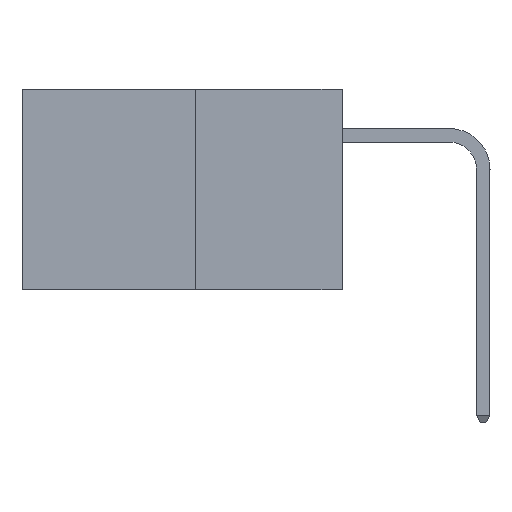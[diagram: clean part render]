
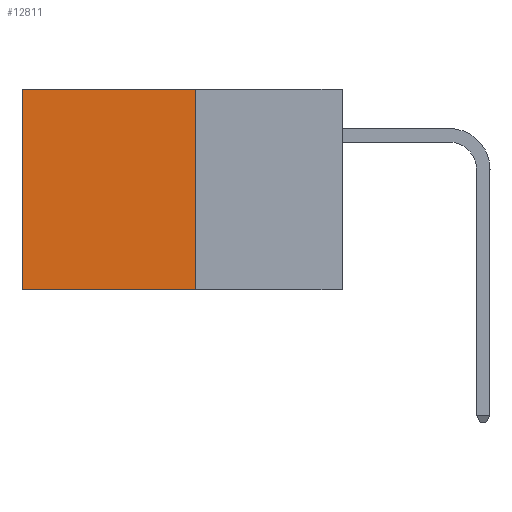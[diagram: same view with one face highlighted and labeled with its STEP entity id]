
A CAD part, left-side view. The second image highlights one B-rep face of the part: STEP entity #12811.
In plain terms, the highlighted planar face has unit normal (-1, 0, 0).
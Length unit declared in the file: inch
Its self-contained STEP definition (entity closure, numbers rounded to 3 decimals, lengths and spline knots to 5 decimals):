
#81 = VERTEX_POINT ( 'NONE', #2989 ) ;
#123 = EDGE_CURVE ( 'NONE', #5820, #247, #1685, .T. ) ;
#197 = CARTESIAN_POINT ( 'NONE',  ( 0.277, 0.59, -0.37 ) ) ;
#247 = VERTEX_POINT ( 'NONE', #4695 ) ;
#1388 = PLANE ( 'NONE',  #12118 ) ;
#1685 = LINE ( 'NONE', #8712, #4785 ) ;
#2610 = DIRECTION ( 'NONE',  ( 0., 0., -1. ) ) ;
#2716 = VECTOR ( 'NONE', #12440, 39.37008 ) ;
#2989 = CARTESIAN_POINT ( 'NONE',  ( 0.277, 0.59, 0. ) ) ;
#3419 = CARTESIAN_POINT ( 'NONE',  ( 0.277, 0.27, -0.37 ) ) ;
#4319 = EDGE_CURVE ( 'NONE', #13205, #81, #5740, .T. ) ;
#4546 = CARTESIAN_POINT ( 'NONE',  ( 0.277, 0.27, 0. ) ) ;
#4695 = CARTESIAN_POINT ( 'NONE',  ( 0.277, 0.59, -0.37 ) ) ;
#4785 = VECTOR ( 'NONE', #13784, 39.37008 ) ;
#5039 = VECTOR ( 'NONE', #7945, 39.37008 ) ;
#5740 = LINE ( 'NONE', #4546, #5039 ) ;
#5751 = LINE ( 'NONE', #3419, #2716 ) ;
#5820 = VERTEX_POINT ( 'NONE', #7116 ) ;
#5882 = ORIENTED_EDGE ( 'NONE', *, *, #11241, .F. ) ;
#6765 = ORIENTED_EDGE ( 'NONE', *, *, #123, .F. ) ;
#7116 = CARTESIAN_POINT ( 'NONE',  ( 0.277, 0.27, -0.37 ) ) ;
#7132 = CARTESIAN_POINT ( 'NONE',  ( 0.277, 0.27, -0.37 ) ) ;
#7712 = ORIENTED_EDGE ( 'NONE', *, *, #12129, .T. ) ;
#7945 = DIRECTION ( 'NONE',  ( 0., 1., 0. ) ) ;
#8011 = LINE ( 'NONE', #197, #14291 ) ;
#8712 = CARTESIAN_POINT ( 'NONE',  ( 0.277, 0.27, -0.37 ) ) ;
#9398 = DIRECTION ( 'NONE',  ( 1., 0., 0. ) ) ;
#9446 = DIRECTION ( 'NONE',  ( 0., 0., -1. ) ) ;
#9824 = EDGE_LOOP ( 'NONE', ( #7712, #6765, #5882, #14040 ) ) ;
#11241 = EDGE_CURVE ( 'NONE', #13205, #5820, #5751, .T. ) ;
#12118 = AXIS2_PLACEMENT_3D ( 'NONE', #7132, #9398, #2610 ) ;
#12129 = EDGE_CURVE ( 'NONE', #81, #247, #8011, .T. ) ;
#12440 = DIRECTION ( 'NONE',  ( 0., 0., -1. ) ) ;
#12811 = ADVANCED_FACE ( 'NONE', ( #13438 ), #1388, .F. ) ;
#13205 = VERTEX_POINT ( 'NONE', #13381 ) ;
#13381 = CARTESIAN_POINT ( 'NONE',  ( 0.277, 0.27, 0. ) ) ;
#13438 = FACE_OUTER_BOUND ( 'NONE', #9824, .T. ) ;
#13784 = DIRECTION ( 'NONE',  ( 0., 1., 0. ) ) ;
#14040 = ORIENTED_EDGE ( 'NONE', *, *, #4319, .T. ) ;
#14291 = VECTOR ( 'NONE', #9446, 39.37008 ) ;
